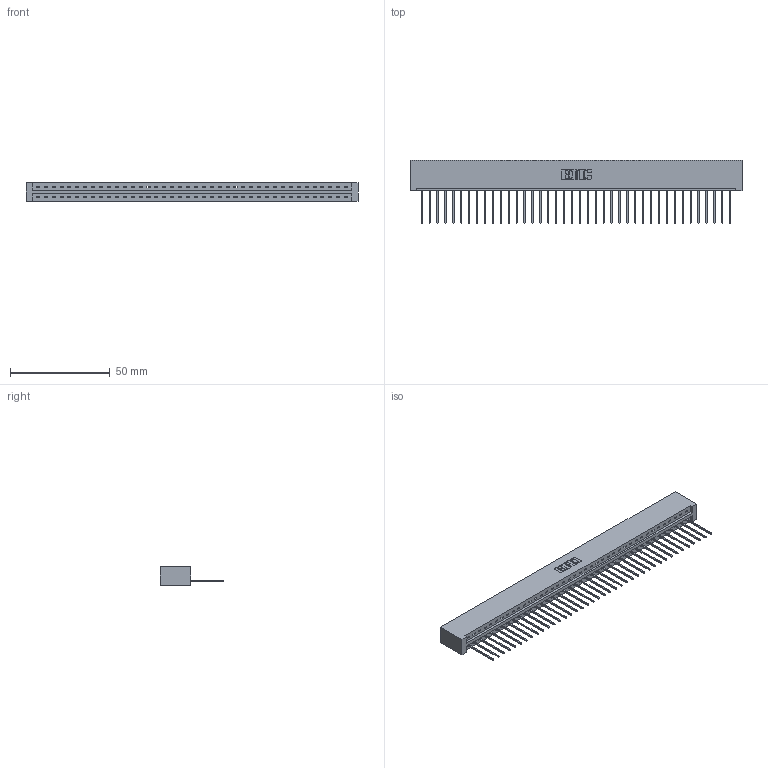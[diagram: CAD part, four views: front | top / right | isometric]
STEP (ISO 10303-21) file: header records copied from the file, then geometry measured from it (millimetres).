
FILE_DESCRIPTION (( 'STEP AP203' ), '1' );
FILE_NAME ('387-040-542-101.STEP', '2019-10-04T18:56:15', ( '' ), ( '' ), 'SwSTEP 2.0', 'SolidWorks 2016', '' );
FILE_SCHEMA (( 'CONFIG_CONTROL_DESIGN' ));
Length unit declared in the file: inch
Products named in the file (3): 387-040-542-101; 345-292-001_345-293-142; 337 Part_No Mounting Lugs
Assembly tree (41 placements, depth 2):
  387-040-542-101
    337 Part_No Mounting Lugs
    345-292-001_345-293-142  x40
Bounding box: 166.37 x 31.63 x 9.4 mm (x, y, z)
Volume: 18094 mm3; surface area: 19253.2 mm2
Topology: 41 solids, 41 shells, 2586 faces, 7807 edges, 5150 vertices
Faces by surface type: plane 1906, cylinder 680
Entity records: 29733 total; most frequent: CARTESIAN_POINT 5186, ORIENTED_EDGE 5162, DIRECTION 4361, EDGE_CURVE 2581, LINE 2461, VECTOR 2461, VERTEX_POINT 1718, AXIS2_PLACEMENT_3D 950
